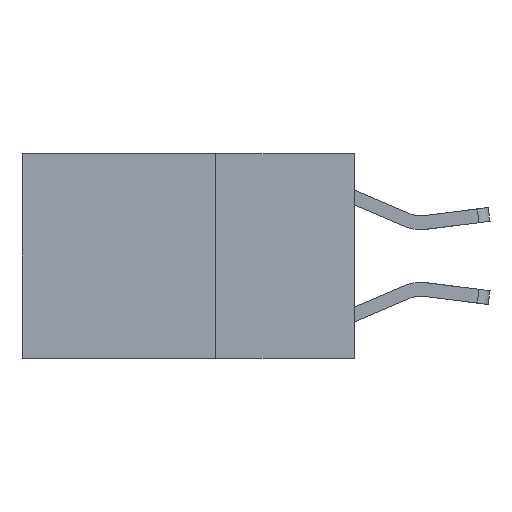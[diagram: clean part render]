
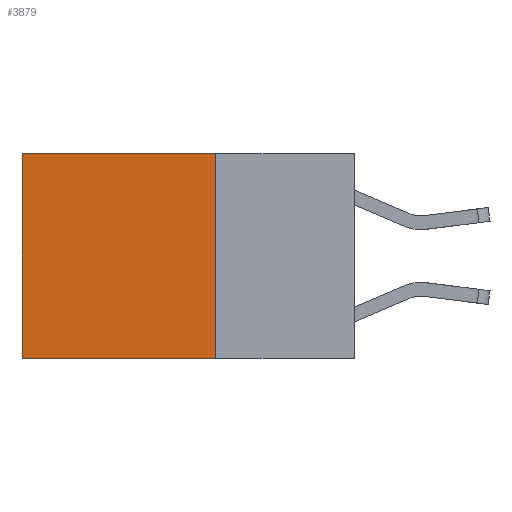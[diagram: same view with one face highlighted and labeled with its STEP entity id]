
A CAD part, left-side view. The second image highlights one B-rep face of the part: STEP entity #3879.
In plain terms, the highlighted planar face has unit normal (-1, 0, 0).
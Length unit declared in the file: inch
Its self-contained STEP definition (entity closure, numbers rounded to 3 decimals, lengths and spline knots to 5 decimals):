
#715 = DIRECTION ( 'NONE',  ( 0., 1., 0. ) ) ;
#1401 = DIRECTION ( 'NONE',  ( 0., 0., -1. ) ) ;
#1479 = DIRECTION ( 'NONE',  ( 0., 0., -1. ) ) ;
#1504 = LINE ( 'NONE', #8143, #10150 ) ;
#1563 = LINE ( 'NONE', #2385, #8421 ) ;
#1708 = VERTEX_POINT ( 'NONE', #8580 ) ;
#2277 = CARTESIAN_POINT ( 'NONE',  ( 0.2625, 0.25, 0. ) ) ;
#2385 = CARTESIAN_POINT ( 'NONE',  ( 0.2625, 0.25, -0.37 ) ) ;
#2518 = DIRECTION ( 'NONE',  ( 0., 0., -1. ) ) ;
#3026 = VECTOR ( 'NONE', #1479, 39.37008 ) ;
#3840 = CARTESIAN_POINT ( 'NONE',  ( 0.2625, 0.6, -0.37 ) ) ;
#3879 = ADVANCED_FACE ( 'NONE', ( #5873 ), #6665, .F. ) ;
#4234 = CARTESIAN_POINT ( 'NONE',  ( 0.2625, 0.25, 0. ) ) ;
#4240 = ORIENTED_EDGE ( 'NONE', *, *, #6706, .F. ) ;
#5572 = DIRECTION ( 'NONE',  ( 0., 1., 0. ) ) ;
#5870 = VERTEX_POINT ( 'NONE', #2277 ) ;
#5873 = FACE_OUTER_BOUND ( 'NONE', #6405, .T. ) ;
#6405 = EDGE_LOOP ( 'NONE', ( #6507, #4240, #9427, #10153 ) ) ;
#6507 = ORIENTED_EDGE ( 'NONE', *, *, #6761, .T. ) ;
#6665 = PLANE ( 'NONE',  #7339 ) ;
#6706 = EDGE_CURVE ( 'NONE', #10510, #7883, #1563, .T. ) ;
#6761 = EDGE_CURVE ( 'NONE', #1708, #7883, #1504, .T. ) ;
#7339 = AXIS2_PLACEMENT_3D ( 'NONE', #4234, #10663, #2518 ) ;
#7844 = LINE ( 'NONE', #9787, #9399 ) ;
#7883 = VERTEX_POINT ( 'NONE', #3840 ) ;
#8143 = CARTESIAN_POINT ( 'NONE',  ( 0.2625, 0.6, 0. ) ) ;
#8232 = CARTESIAN_POINT ( 'NONE',  ( 0.2625, 0.25, 0. ) ) ;
#8421 = VECTOR ( 'NONE', #5572, 39.37008 ) ;
#8580 = CARTESIAN_POINT ( 'NONE',  ( 0.2625, 0.6, 0. ) ) ;
#9399 = VECTOR ( 'NONE', #715, 39.37008 ) ;
#9427 = ORIENTED_EDGE ( 'NONE', *, *, #10279, .F. ) ;
#9463 = CARTESIAN_POINT ( 'NONE',  ( 0.2625, 0.25, -0.37 ) ) ;
#9787 = CARTESIAN_POINT ( 'NONE',  ( 0.2625, 0.25, 0. ) ) ;
#9852 = LINE ( 'NONE', #8232, #3026 ) ;
#10150 = VECTOR ( 'NONE', #1401, 39.37008 ) ;
#10153 = ORIENTED_EDGE ( 'NONE', *, *, #10589, .T. ) ;
#10279 = EDGE_CURVE ( 'NONE', #5870, #10510, #9852, .T. ) ;
#10510 = VERTEX_POINT ( 'NONE', #9463 ) ;
#10589 = EDGE_CURVE ( 'NONE', #5870, #1708, #7844, .T. ) ;
#10663 = DIRECTION ( 'NONE',  ( 1., 0., 0. ) ) ;
